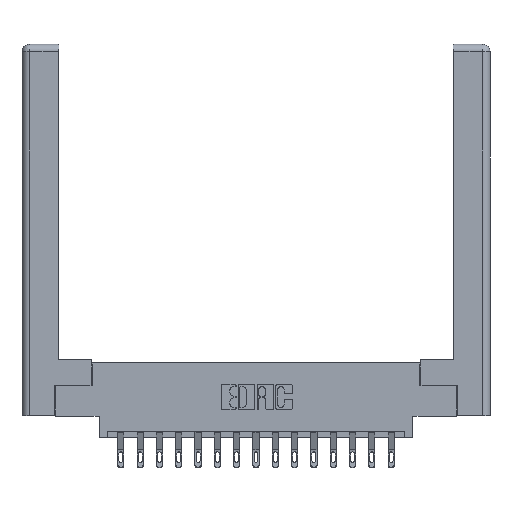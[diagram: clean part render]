
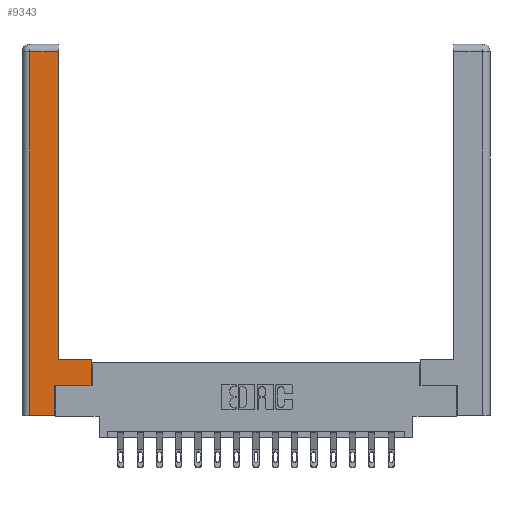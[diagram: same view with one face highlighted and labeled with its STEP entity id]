
A CAD part, top view. The second image highlights one B-rep face of the part: STEP entity #9343.
In plain terms, the highlighted planar face has unit normal (0, 0, 1).
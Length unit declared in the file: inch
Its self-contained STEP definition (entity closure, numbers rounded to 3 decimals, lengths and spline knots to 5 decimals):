
#851 = ORIENTED_EDGE ( 'NONE', *, *, #3427, .T. ) ;
#922 = AXIS2_PLACEMENT_3D ( 'NONE', #1417, #11247, #16838 ) ;
#1165 = VERTEX_POINT ( 'NONE', #14965 ) ;
#1417 = CARTESIAN_POINT ( 'NONE',  ( 0., 0., 0. ) ) ;
#2001 = LINE ( 'NONE', #14198, #14392 ) ;
#2245 = DIRECTION ( 'NONE',  ( 1., 0., 0. ) ) ;
#2248 = VECTOR ( 'NONE', #6236, 39.37008 ) ;
#2644 = CARTESIAN_POINT ( 'NONE',  ( 0.0615, 0., 0. ) ) ;
#3144 = EDGE_CURVE ( 'NONE', #17892, #6618, #8883, .T. ) ;
#3320 = VECTOR ( 'NONE', #11343, 39.37008 ) ;
#3427 = EDGE_CURVE ( 'NONE', #16762, #17892, #13521, .T. ) ;
#4002 = EDGE_CURVE ( 'NONE', #6618, #4030, #2001, .T. ) ;
#4030 = VERTEX_POINT ( 'NONE', #15808 ) ;
#4224 = ORIENTED_EDGE ( 'NONE', *, *, #8104, .T. ) ;
#4661 = ORIENTED_EDGE ( 'NONE', *, *, #9891, .T. ) ;
#4946 = VECTOR ( 'NONE', #2245, 39.37008 ) ;
#4965 = CARTESIAN_POINT ( 'NONE',  ( 0.265, 0., 0. ) ) ;
#5392 = VERTEX_POINT ( 'NONE', #9665 ) ;
#5489 = CARTESIAN_POINT ( 'NONE',  ( 0.265, 0.245, 0. ) ) ;
#6104 = ORIENTED_EDGE ( 'NONE', *, *, #10812, .T. ) ;
#6236 = DIRECTION ( 'NONE',  ( -1., 0., 0. ) ) ;
#6337 = CARTESIAN_POINT ( 'NONE',  ( 0.565, 0.245, 0. ) ) ;
#6618 = VERTEX_POINT ( 'NONE', #10617 ) ;
#6932 = ORIENTED_EDGE ( 'NONE', *, *, #3144, .T. ) ;
#8104 = EDGE_CURVE ( 'NONE', #17978, #1165, #18186, .T. ) ;
#8220 = CARTESIAN_POINT ( 'NONE',  ( 0.565, 0.45, 0. ) ) ;
#8712 = CARTESIAN_POINT ( 'NONE',  ( 0.0615, 0., 0. ) ) ;
#8853 = VECTOR ( 'NONE', #16557, 39.37008 ) ;
#8883 = LINE ( 'NONE', #10508, #2248 ) ;
#9343 = ADVANCED_FACE ( 'NONE', ( #13524 ), #18049, .F. ) ;
#9422 = ORIENTED_EDGE ( 'NONE', *, *, #13427, .T. ) ;
#9577 = ORIENTED_EDGE ( 'NONE', *, *, #10266, .T. ) ;
#9665 = CARTESIAN_POINT ( 'NONE',  ( 0.265, 0.245, 0. ) ) ;
#9891 = EDGE_CURVE ( 'NONE', #5392, #16762, #11726, .T. ) ;
#9898 = DIRECTION ( 'NONE',  ( 0., 1., 0. ) ) ;
#10266 = EDGE_CURVE ( 'NONE', #17151, #17978, #11918, .T. ) ;
#10508 = CARTESIAN_POINT ( 'NONE',  ( 0.295, 0.45, 0. ) ) ;
#10617 = CARTESIAN_POINT ( 'NONE',  ( 0.295, 0.45, 0. ) ) ;
#10667 = CARTESIAN_POINT ( 'NONE',  ( 0.0615, 2.94, 0. ) ) ;
#10812 = EDGE_CURVE ( 'NONE', #4030, #17151, #15709, .T. ) ;
#11247 = DIRECTION ( 'NONE',  ( 0., 0., -1. ) ) ;
#11343 = DIRECTION ( 'NONE',  ( 0., -1., 0. ) ) ;
#11726 = LINE ( 'NONE', #17853, #15066 ) ;
#11918 = LINE ( 'NONE', #2644, #3320 ) ;
#12889 = DIRECTION ( 'NONE',  ( 0., 1., 0. ) ) ;
#13427 = EDGE_CURVE ( 'NONE', #1165, #5392, #17992, .T. ) ;
#13521 = LINE ( 'NONE', #14282, #14623 ) ;
#13524 = FACE_OUTER_BOUND ( 'NONE', #13963, .T. ) ;
#13682 = DIRECTION ( 'NONE',  ( 1., 0., 0. ) ) ;
#13963 = EDGE_LOOP ( 'NONE', ( #13997, #6104, #9577, #4224, #9422, #4661, #851, #6932 ) ) ;
#13997 = ORIENTED_EDGE ( 'NONE', *, *, #4002, .T. ) ;
#14198 = CARTESIAN_POINT ( 'NONE',  ( 0.295, 3., 0. ) ) ;
#14214 = DIRECTION ( 'NONE',  ( 0., 1., 0. ) ) ;
#14282 = CARTESIAN_POINT ( 'NONE',  ( 0.565, 0.45, 0. ) ) ;
#14392 = VECTOR ( 'NONE', #12889, 39.37008 ) ;
#14623 = VECTOR ( 'NONE', #14214, 39.37008 ) ;
#14965 = CARTESIAN_POINT ( 'NONE',  ( 0.265, 0., 0. ) ) ;
#15066 = VECTOR ( 'NONE', #13682, 39.37008 ) ;
#15155 = VECTOR ( 'NONE', #9898, 39.37008 ) ;
#15709 = LINE ( 'NONE', #10667, #8853 ) ;
#15808 = CARTESIAN_POINT ( 'NONE',  ( 0.295, 2.94, 0. ) ) ;
#16557 = DIRECTION ( 'NONE',  ( -1., 0., 0. ) ) ;
#16762 = VERTEX_POINT ( 'NONE', #6337 ) ;
#16838 = DIRECTION ( 'NONE',  ( -1., 0., 0. ) ) ;
#17024 = CARTESIAN_POINT ( 'NONE',  ( 0.0615, 2.94, 0. ) ) ;
#17151 = VERTEX_POINT ( 'NONE', #17024 ) ;
#17853 = CARTESIAN_POINT ( 'NONE',  ( 0.565, 0.245, 0. ) ) ;
#17892 = VERTEX_POINT ( 'NONE', #8220 ) ;
#17978 = VERTEX_POINT ( 'NONE', #8712 ) ;
#17992 = LINE ( 'NONE', #5489, #15155 ) ;
#18049 = PLANE ( 'NONE',  #922 ) ;
#18186 = LINE ( 'NONE', #4965, #4946 ) ;
